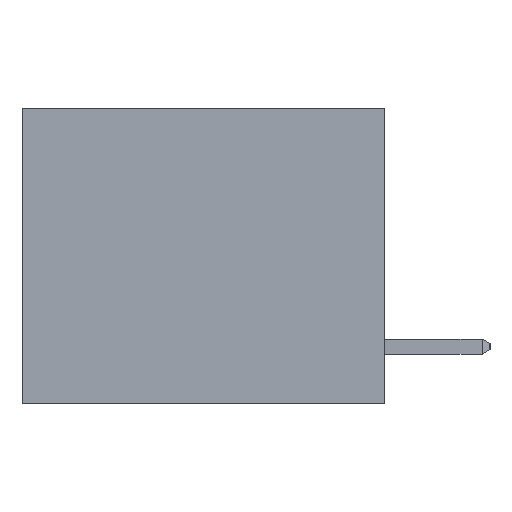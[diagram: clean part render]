
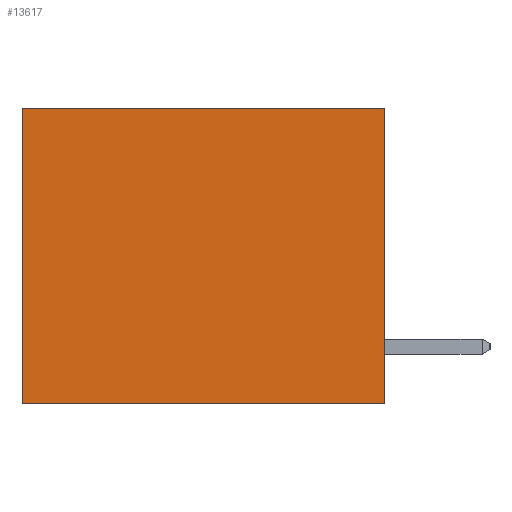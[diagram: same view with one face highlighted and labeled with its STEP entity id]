
A CAD part, left-side view. The second image highlights one B-rep face of the part: STEP entity #13617.
In plain terms, the highlighted planar face has unit normal (-1, 0, 0).
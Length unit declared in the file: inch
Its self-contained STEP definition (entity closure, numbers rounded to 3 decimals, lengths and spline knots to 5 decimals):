
#551 = VERTEX_POINT ( 'NONE', #14212 ) ;
#609 = ORIENTED_EDGE ( 'NONE', *, *, #2182, .T. ) ;
#1080 = VERTEX_POINT ( 'NONE', #13388 ) ;
#1327 = CARTESIAN_POINT ( 'NONE',  ( 0.3165, 0., 0. ) ) ;
#2182 = EDGE_CURVE ( 'NONE', #551, #1080, #11539, .T. ) ;
#3162 = DIRECTION ( 'NONE',  ( 0., 1., 0. ) ) ;
#3823 = VECTOR ( 'NONE', #8117, 39.37008 ) ;
#5730 = CARTESIAN_POINT ( 'NONE',  ( 0.3165, 0., 0. ) ) ;
#6811 = CARTESIAN_POINT ( 'NONE',  ( 0.3165, 0., -0.49 ) ) ;
#7015 = DIRECTION ( 'NONE',  ( 1., 0., 0. ) ) ;
#7058 = EDGE_LOOP ( 'NONE', ( #609, #18354, #18518, #9438 ) ) ;
#8117 = DIRECTION ( 'NONE',  ( 0., 0., -1. ) ) ;
#9228 = LINE ( 'NONE', #13480, #3823 ) ;
#9438 = ORIENTED_EDGE ( 'NONE', *, *, #11009, .T. ) ;
#9930 = CARTESIAN_POINT ( 'NONE',  ( 0.3165, 0., -0.49 ) ) ;
#10289 = VECTOR ( 'NONE', #15142, 39.37008 ) ;
#10849 = VERTEX_POINT ( 'NONE', #5730 ) ;
#11009 = EDGE_CURVE ( 'NONE', #10849, #551, #20726, .T. ) ;
#11539 = LINE ( 'NONE', #21528, #22891 ) ;
#11798 = FACE_OUTER_BOUND ( 'NONE', #7058, .T. ) ;
#13048 = DIRECTION ( 'NONE',  ( 0., 0., -1. ) ) ;
#13347 = VECTOR ( 'NONE', #3162, 39.37008 ) ;
#13388 = CARTESIAN_POINT ( 'NONE',  ( 0.3165, 0.6, -0.49 ) ) ;
#13480 = CARTESIAN_POINT ( 'NONE',  ( 0.3165, 0., -0.49 ) ) ;
#13617 = ADVANCED_FACE ( 'NONE', ( #11798 ), #17886, .F. ) ;
#14212 = CARTESIAN_POINT ( 'NONE',  ( 0.3165, 0.6, 0. ) ) ;
#15142 = DIRECTION ( 'NONE',  ( 0., 1., 0. ) ) ;
#15258 = EDGE_CURVE ( 'NONE', #10849, #22463, #9228, .T. ) ;
#16306 = CARTESIAN_POINT ( 'NONE',  ( 0.3165, 0., -0.49 ) ) ;
#17886 = PLANE ( 'NONE',  #19284 ) ;
#17964 = DIRECTION ( 'NONE',  ( 0., 0., -1. ) ) ;
#18354 = ORIENTED_EDGE ( 'NONE', *, *, #21100, .F. ) ;
#18518 = ORIENTED_EDGE ( 'NONE', *, *, #15258, .F. ) ;
#19113 = LINE ( 'NONE', #6811, #10289 ) ;
#19284 = AXIS2_PLACEMENT_3D ( 'NONE', #16306, #7015, #17964 ) ;
#20726 = LINE ( 'NONE', #1327, #13347 ) ;
#21100 = EDGE_CURVE ( 'NONE', #22463, #1080, #19113, .T. ) ;
#21528 = CARTESIAN_POINT ( 'NONE',  ( 0.3165, 0.6, -0.49 ) ) ;
#22463 = VERTEX_POINT ( 'NONE', #9930 ) ;
#22891 = VECTOR ( 'NONE', #13048, 39.37008 ) ;
